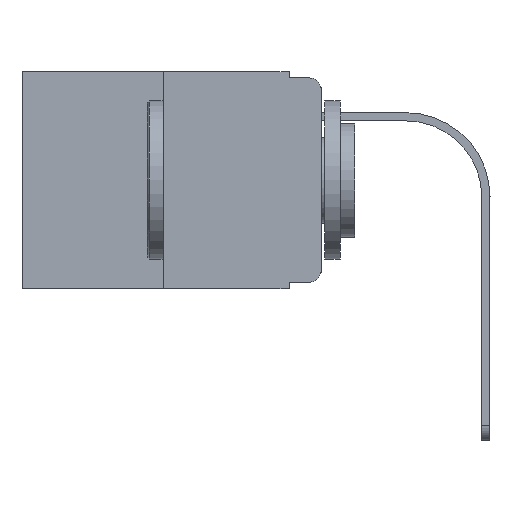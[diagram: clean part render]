
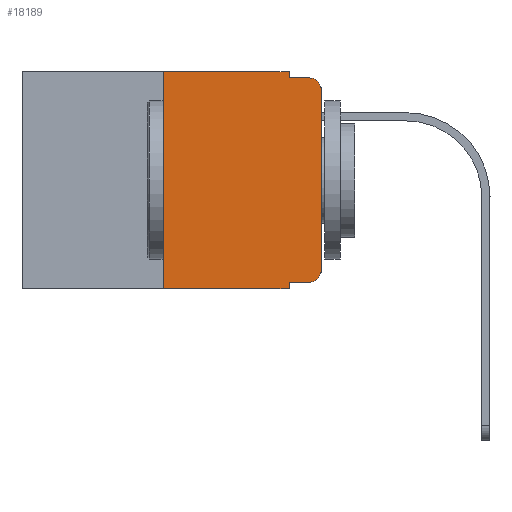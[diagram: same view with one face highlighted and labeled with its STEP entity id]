
A CAD part, left-side view. The second image highlights one B-rep face of the part: STEP entity #18189.
In plain terms, the highlighted planar face has unit normal (-1, 0, 0).
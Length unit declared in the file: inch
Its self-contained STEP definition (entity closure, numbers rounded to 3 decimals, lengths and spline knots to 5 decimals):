
#77 = VECTOR ( 'NONE', #12579, 39.37008 ) ;
#676 = DIRECTION ( 'NONE',  ( 0., 0., 1. ) ) ;
#1406 = CARTESIAN_POINT ( 'NONE',  ( 0., 0.25, 0. ) ) ;
#1707 = CARTESIAN_POINT ( 'NONE',  ( 0., 0.473, 0. ) ) ;
#2117 = DIRECTION ( 'NONE',  ( 0., 0., -1. ) ) ;
#2654 = VECTOR ( 'NONE', #8393, 39.37008 ) ;
#2732 = CARTESIAN_POINT ( 'NONE',  ( 0., 0.051, -0.333 ) ) ;
#2783 = ORIENTED_EDGE ( 'NONE', *, *, #20477, .F. ) ;
#2806 = VERTEX_POINT ( 'NONE', #18890 ) ;
#2891 = EDGE_CURVE ( 'NONE', #15358, #13822, #4531, .T. ) ;
#3065 = CARTESIAN_POINT ( 'NONE',  ( 0., 0., -0.313 ) ) ;
#3744 = CIRCLE ( 'NONE', #10701, 0.02 ) ;
#3750 = DIRECTION ( 'NONE',  ( 0., -1., 0. ) ) ;
#3789 = ORIENTED_EDGE ( 'NONE', *, *, #9204, .T. ) ;
#3877 = ORIENTED_EDGE ( 'NONE', *, *, #9660, .T. ) ;
#4522 = CARTESIAN_POINT ( 'NONE',  ( 0., 0.25, 0. ) ) ;
#4531 = CIRCLE ( 'NONE', #12228, 0.02 ) ;
#4708 = VECTOR ( 'NONE', #3750, 39.37008 ) ;
#4741 = CARTESIAN_POINT ( 'NONE',  ( 0., 0.02, -0.313 ) ) ;
#4854 = VECTOR ( 'NONE', #676, 39.37008 ) ;
#5002 = ORIENTED_EDGE ( 'NONE', *, *, #8855, .F. ) ;
#5074 = DIRECTION ( 'NONE',  ( 1., 0., 0. ) ) ;
#5224 = VERTEX_POINT ( 'NONE', #13850 ) ;
#5356 = VERTEX_POINT ( 'NONE', #2732 ) ;
#5773 = EDGE_CURVE ( 'NONE', #7557, #2806, #16223, .T. ) ;
#5866 = VECTOR ( 'NONE', #11514, 39.37008 ) ;
#6287 = ORIENTED_EDGE ( 'NONE', *, *, #7120, .F. ) ;
#6451 = DIRECTION ( 'NONE',  ( 0., -1., 0. ) ) ;
#6819 = DIRECTION ( 'NONE',  ( 0., 0., -1. ) ) ;
#7024 = LINE ( 'NONE', #13867, #2654 ) ;
#7120 = EDGE_CURVE ( 'NONE', #2806, #10897, #22039, .T. ) ;
#7530 = CARTESIAN_POINT ( 'NONE',  ( 0., 0.051, 0. ) ) ;
#7557 = VERTEX_POINT ( 'NONE', #19685 ) ;
#7837 = EDGE_CURVE ( 'NONE', #17950, #9627, #13239, .T. ) ;
#7845 = CARTESIAN_POINT ( 'NONE',  ( 0., 0.02, -0.333 ) ) ;
#7911 = ORIENTED_EDGE ( 'NONE', *, *, #2891, .T. ) ;
#8393 = DIRECTION ( 'NONE',  ( 0., -1., 0. ) ) ;
#8855 = EDGE_CURVE ( 'NONE', #9627, #7557, #17475, .T. ) ;
#8884 = PLANE ( 'NONE',  #22188 ) ;
#9053 = LINE ( 'NONE', #19625, #15016 ) ;
#9094 = EDGE_CURVE ( 'NONE', #13822, #13972, #11100, .T. ) ;
#9204 = EDGE_CURVE ( 'NONE', #13972, #10897, #3744, .T. ) ;
#9627 = VERTEX_POINT ( 'NONE', #1406 ) ;
#9660 = EDGE_CURVE ( 'NONE', #5356, #15358, #7024, .T. ) ;
#9998 = CARTESIAN_POINT ( 'NONE',  ( 0., 0.051, -0.01 ) ) ;
#10074 = ORIENTED_EDGE ( 'NONE', *, *, #5773, .F. ) ;
#10701 = AXIS2_PLACEMENT_3D ( 'NONE', #17120, #20274, #11884 ) ;
#10897 = VERTEX_POINT ( 'NONE', #20893 ) ;
#11100 = LINE ( 'NONE', #12695, #4854 ) ;
#11514 = DIRECTION ( 'NONE',  ( 0., 0., 1. ) ) ;
#11862 = DIRECTION ( 'NONE',  ( -1., 0., 0. ) ) ;
#11884 = DIRECTION ( 'NONE',  ( 0., 0., -1. ) ) ;
#12228 = AXIS2_PLACEMENT_3D ( 'NONE', #4741, #11862, #15184 ) ;
#12579 = DIRECTION ( 'NONE',  ( 0., -1., 0. ) ) ;
#12695 = CARTESIAN_POINT ( 'NONE',  ( 0., 0., 0. ) ) ;
#13059 = ORIENTED_EDGE ( 'NONE', *, *, #9094, .T. ) ;
#13239 = LINE ( 'NONE', #4522, #5866 ) ;
#13822 = VERTEX_POINT ( 'NONE', #3065 ) ;
#13850 = CARTESIAN_POINT ( 'NONE',  ( 0., 0.051, -0.343 ) ) ;
#13867 = CARTESIAN_POINT ( 'NONE',  ( 0., 0.051, -0.333 ) ) ;
#13928 = CARTESIAN_POINT ( 'NONE',  ( 0., 0., -0.03 ) ) ;
#13972 = VERTEX_POINT ( 'NONE', #13928 ) ;
#14165 = LINE ( 'NONE', #19260, #77 ) ;
#14730 = CARTESIAN_POINT ( 'NONE',  ( 0., 0.25, -0.343 ) ) ;
#15016 = VECTOR ( 'NONE', #17398, 39.37008 ) ;
#15184 = DIRECTION ( 'NONE',  ( 0., 0., -1. ) ) ;
#15358 = VERTEX_POINT ( 'NONE', #7845 ) ;
#15851 = CARTESIAN_POINT ( 'NONE',  ( 0., 0.473, 0. ) ) ;
#16069 = ORIENTED_EDGE ( 'NONE', *, *, #7837, .F. ) ;
#16223 = LINE ( 'NONE', #7530, #16836 ) ;
#16836 = VECTOR ( 'NONE', #2117, 39.37008 ) ;
#17120 = CARTESIAN_POINT ( 'NONE',  ( 0., 0.02, -0.03 ) ) ;
#17398 = DIRECTION ( 'NONE',  ( 0., 0., -1. ) ) ;
#17475 = LINE ( 'NONE', #1707, #4708 ) ;
#17879 = EDGE_LOOP ( 'NONE', ( #13059, #3789, #6287, #10074, #5002, #16069, #21425, #2783, #3877, #7911 ) ) ;
#17950 = VERTEX_POINT ( 'NONE', #14730 ) ;
#18189 = ADVANCED_FACE ( 'NONE', ( #22412 ), #8884, .F. ) ;
#18238 = VECTOR ( 'NONE', #6451, 39.37008 ) ;
#18890 = CARTESIAN_POINT ( 'NONE',  ( 0., 0.051, -0.01 ) ) ;
#19260 = CARTESIAN_POINT ( 'NONE',  ( 0., 0.473, -0.343 ) ) ;
#19625 = CARTESIAN_POINT ( 'NONE',  ( 0., 0.051, 0. ) ) ;
#19685 = CARTESIAN_POINT ( 'NONE',  ( 0., 0.051, 0. ) ) ;
#20274 = DIRECTION ( 'NONE',  ( -1., 0., 0. ) ) ;
#20477 = EDGE_CURVE ( 'NONE', #5356, #5224, #9053, .T. ) ;
#20893 = CARTESIAN_POINT ( 'NONE',  ( 0., 0.02, -0.01 ) ) ;
#21425 = ORIENTED_EDGE ( 'NONE', *, *, #22097, .T. ) ;
#22039 = LINE ( 'NONE', #9998, #18238 ) ;
#22097 = EDGE_CURVE ( 'NONE', #17950, #5224, #14165, .T. ) ;
#22188 = AXIS2_PLACEMENT_3D ( 'NONE', #15851, #5074, #6819 ) ;
#22412 = FACE_OUTER_BOUND ( 'NONE', #17879, .T. ) ;
